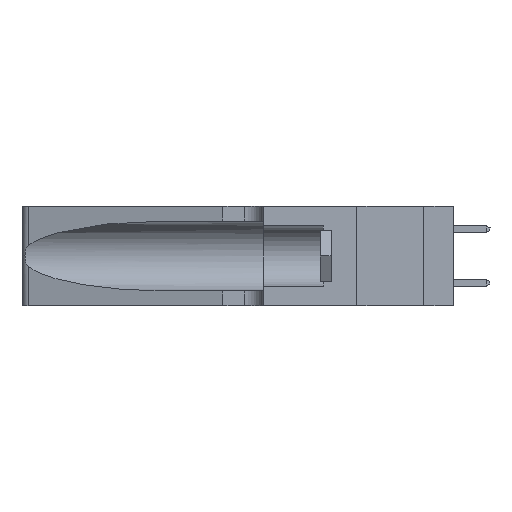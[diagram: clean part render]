
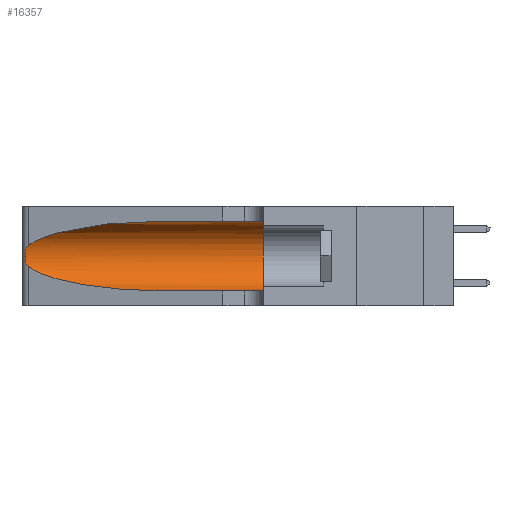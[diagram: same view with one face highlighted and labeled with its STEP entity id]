
A CAD part, left-side view. The second image highlights one B-rep face of the part: STEP entity #16357.
In plain terms, the highlighted cylindrical face has radius 3.308 mm (diameter 6.617 mm), a partial arc.
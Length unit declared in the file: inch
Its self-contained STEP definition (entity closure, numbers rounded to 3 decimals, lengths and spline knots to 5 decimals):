
#286 = EDGE_CURVE ( 'NONE', #29109, #21350, #24931, .T. ) ;
#287 = LINE ( 'NONE', #7383, #27087 ) ;
#943 = CARTESIAN_POINT ( 'NONE',  ( 0.25639, 1.23184, 0.21858 ) ) ;
#1372 = EDGE_CURVE ( 'NONE', #21755, #21350, #287, .T. ) ;
#1993 = EDGE_LOOP ( 'NONE', ( #25750, #42320, #4675, #16165, #11225, #16624 ) ) ;
#2221 = DIRECTION ( 'NONE',  ( 0., 1., 0. ) ) ;
#4498 = CARTESIAN_POINT ( 'NONE',  ( 0.25854, 1.2359, 0.20912 ) ) ;
#4675 = ORIENTED_EDGE ( 'NONE', *, *, #16032, .T. ) ;
#4816 = B_SPLINE_CURVE_WITH_KNOTS ( 'NONE', 3,
 ( #42615, #28719, #943, #25393, #4498, #28867, #8013, #32315, #11549, #35761, #15066, #39269, #18585, #42770 ),
 .UNSPECIFIED., .F., .F.,
 ( 4, 2, 2, 2, 2, 2, 4 ),
 ( 0., 0.00027, 0.00053, 0.00107, 0.0016, 0.00187, 0.00214 ),
 .UNSPECIFIED. ) ;
#6374 = AXIS2_PLACEMENT_3D ( 'NONE', #21195, #38370, #27834 ) ;
#7383 = CARTESIAN_POINT ( 'NONE',  ( 0.1305, 1.61858, 0.05475 ) ) ;
#7830 = CARTESIAN_POINT ( 'NONE',  ( 0.1305, 0.72297, 0.31525 ) ) ;
#8013 = CARTESIAN_POINT ( 'NONE',  ( 0.26075, 1.23896, 0.19203 ) ) ;
#8041 = CARTESIAN_POINT ( 'NONE',  ( 0.25487, 1.22718, 0.22369 ) ) ;
#8818 = DIRECTION ( 'NONE',  ( 0., -1., 0. ) ) ;
#9272 = CARTESIAN_POINT ( 'NONE',  ( 0.2373, 1.15595, 0.08982 ) ) ;
#10670 = CARTESIAN_POINT ( 'NONE',  ( 0.25487, 1.22718, 0.14631 ) ) ;
#10889 = DIRECTION ( 'NONE',  ( 0., -1., 0. ) ) ;
#11225 = ORIENTED_EDGE ( 'NONE', *, *, #286, .F. ) ;
#11549 = CARTESIAN_POINT ( 'NONE',  ( 0.26017, 1.23833, 0.17102 ) ) ;
#12929 =( BOUNDED_CURVE ( )  B_SPLINE_CURVE ( 3, ( #33540, #9272, #30129, #37006 ),
 .UNSPECIFIED., .F., .F. ) 
 B_SPLINE_CURVE_WITH_KNOTS ( ( 4, 4 ),
 ( 3.44316, 4.71239 ),
 .UNSPECIFIED. ) 
 CURVE ( )  GEOMETRIC_REPRESENTATION_ITEM ( )  RATIONAL_B_SPLINE_CURVE ( ( 1., 0.87, 0.87, 1. ) ) 
 REPRESENTATION_ITEM ( '' )  );
#14007 = VERTEX_POINT ( 'NONE', #29374 ) ;
#14712 = CARTESIAN_POINT ( 'NONE',  ( 0.18966, 0.96281, 0.31525 ) ) ;
#14869 = CARTESIAN_POINT ( 'NONE',  ( 0.2373, 1.15595, 0.28018 ) ) ;
#15066 = CARTESIAN_POINT ( 'NONE',  ( 0.25789, 1.23486, 0.15765 ) ) ;
#16032 = EDGE_CURVE ( 'NONE', #18383, #21755, #12929, .T. ) ;
#16052 = CYLINDRICAL_SURFACE ( 'NONE', #6374, 0.13025 ) ;
#16165 = ORIENTED_EDGE ( 'NONE', *, *, #1372, .T. ) ;
#16290 = CARTESIAN_POINT ( 'NONE',  ( 0.1305, 0.35, 0.05475 ) ) ;
#16357 = ADVANCED_FACE ( 'NONE', ( #44721 ), #16052, .F. ) ;
#16624 = ORIENTED_EDGE ( 'NONE', *, *, #16951, .F. ) ;
#16951 = EDGE_CURVE ( 'NONE', #14007, #29109, #19808, .T. ) ;
#17182 = EDGE_CURVE ( 'NONE', #33769, #18383, #4816, .T. ) ;
#18383 = VERTEX_POINT ( 'NONE', #10670 ) ;
#18585 = CARTESIAN_POINT ( 'NONE',  ( 0.25555, 1.22993, 0.14849 ) ) ;
#19808 = LINE ( 'NONE', #31242, #29002 ) ;
#21195 = CARTESIAN_POINT ( 'NONE',  ( 0.1305, 1.61858, 0.185 ) ) ;
#21350 = VERTEX_POINT ( 'NONE', #16290 ) ;
#21716 = EDGE_CURVE ( 'NONE', #14007, #33769, #33739, .T. ) ;
#21755 = VERTEX_POINT ( 'NONE', #42731 ) ;
#23179 = CARTESIAN_POINT ( 'NONE',  ( 0.1305, 0.35, 0.185 ) ) ;
#24931 = CIRCLE ( 'NONE', #41321, 0.13025 ) ;
#25393 = CARTESIAN_POINT ( 'NONE',  ( 0.25787, 1.23484, 0.2124 ) ) ;
#25750 = ORIENTED_EDGE ( 'NONE', *, *, #21716, .T. ) ;
#26646 = DIRECTION ( 'NONE',  ( 0., 0., 1. ) ) ;
#27087 = VECTOR ( 'NONE', #10889, 39.37008 ) ;
#27834 = DIRECTION ( 'NONE',  ( 0., 0., -1. ) ) ;
#28719 = CARTESIAN_POINT ( 'NONE',  ( 0.25555, 1.22994, 0.2215 ) ) ;
#28867 = CARTESIAN_POINT ( 'NONE',  ( 0.26018, 1.23835, 0.19895 ) ) ;
#29002 = VECTOR ( 'NONE', #8818, 39.37008 ) ;
#29109 = VERTEX_POINT ( 'NONE', #42558 ) ;
#29374 = CARTESIAN_POINT ( 'NONE',  ( 0.1305, 0.72297, 0.31525 ) ) ;
#30129 = CARTESIAN_POINT ( 'NONE',  ( 0.18966, 0.96281, 0.05475 ) ) ;
#31242 = CARTESIAN_POINT ( 'NONE',  ( 0.1305, 1.61858, 0.31525 ) ) ;
#32315 = CARTESIAN_POINT ( 'NONE',  ( 0.26075, 1.23896, 0.178 ) ) ;
#33540 = CARTESIAN_POINT ( 'NONE',  ( 0.25487, 1.22718, 0.14631 ) ) ;
#33739 =( BOUNDED_CURVE ( )  B_SPLINE_CURVE ( 3, ( #7830, #14712, #14869, #39083 ),
 .UNSPECIFIED., .F., .F. ) 
 B_SPLINE_CURVE_WITH_KNOTS ( ( 4, 4 ),
 ( 1.5708, 2.84003 ),
 .UNSPECIFIED. ) 
 CURVE ( )  GEOMETRIC_REPRESENTATION_ITEM ( )  RATIONAL_B_SPLINE_CURVE ( ( 1., 0.87, 0.87, 1. ) ) 
 REPRESENTATION_ITEM ( '' )  );
#33769 = VERTEX_POINT ( 'NONE', #8041 ) ;
#35761 = CARTESIAN_POINT ( 'NONE',  ( 0.25856, 1.23593, 0.16098 ) ) ;
#37006 = CARTESIAN_POINT ( 'NONE',  ( 0.1305, 0.72297, 0.05475 ) ) ;
#38370 = DIRECTION ( 'NONE',  ( 0., -1., 0. ) ) ;
#39083 = CARTESIAN_POINT ( 'NONE',  ( 0.25487, 1.22718, 0.22369 ) ) ;
#39269 = CARTESIAN_POINT ( 'NONE',  ( 0.25639, 1.23186, 0.15144 ) ) ;
#41321 = AXIS2_PLACEMENT_3D ( 'NONE', #23179, #2221, #26646 ) ;
#42320 = ORIENTED_EDGE ( 'NONE', *, *, #17182, .T. ) ;
#42558 = CARTESIAN_POINT ( 'NONE',  ( 0.1305, 0.35, 0.31525 ) ) ;
#42615 = CARTESIAN_POINT ( 'NONE',  ( 0.25487, 1.22718, 0.22369 ) ) ;
#42731 = CARTESIAN_POINT ( 'NONE',  ( 0.1305, 0.72297, 0.05475 ) ) ;
#42770 = CARTESIAN_POINT ( 'NONE',  ( 0.25487, 1.22718, 0.14631 ) ) ;
#44721 = FACE_OUTER_BOUND ( 'NONE', #1993, .T. ) ;
